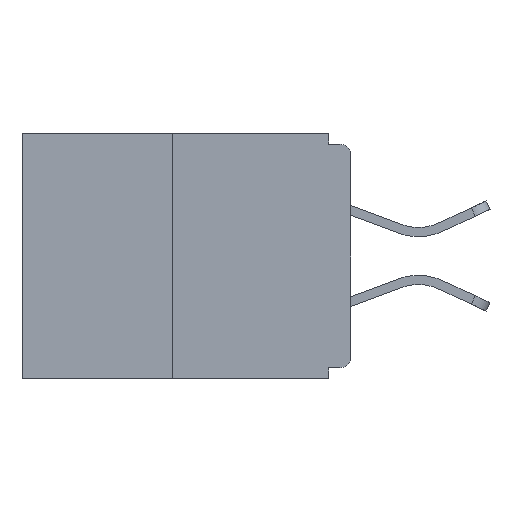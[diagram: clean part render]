
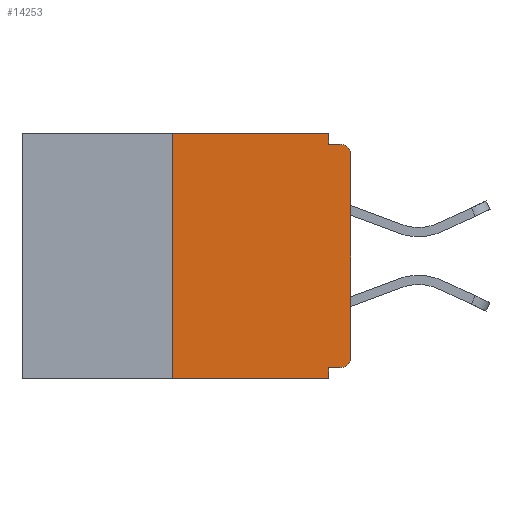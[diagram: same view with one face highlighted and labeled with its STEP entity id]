
A CAD part, left-side view. The second image highlights one B-rep face of the part: STEP entity #14253.
In plain terms, the highlighted planar face has unit normal (-1, 0, 0).
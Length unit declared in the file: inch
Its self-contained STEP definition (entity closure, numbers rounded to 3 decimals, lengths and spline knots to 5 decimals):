
#59 = VERTEX_POINT ( 'NONE', #584 ) ;
#227 = VECTOR ( 'NONE', #20103, 39.37008 ) ;
#247 = DIRECTION ( 'NONE',  ( 0., 0., -1. ) ) ;
#301 = VECTOR ( 'NONE', #11030, 39.37008 ) ;
#584 = CARTESIAN_POINT ( 'NONE',  ( 0., 0., -0.03 ) ) ;
#733 = DIRECTION ( 'NONE',  ( 0., 0., 1. ) ) ;
#843 = VERTEX_POINT ( 'NONE', #1978 ) ;
#1314 = CARTESIAN_POINT ( 'NONE',  ( 0., 0.25, -0.343 ) ) ;
#1721 = DIRECTION ( 'NONE',  ( 0., 0., -1. ) ) ;
#1902 = DIRECTION ( 'NONE',  ( -1., 0., 0. ) ) ;
#1978 = CARTESIAN_POINT ( 'NONE',  ( 0., 0.031, -0.015 ) ) ;
#2137 = VECTOR ( 'NONE', #18872, 39.37008 ) ;
#2547 = VECTOR ( 'NONE', #5426, 39.37008 ) ;
#2620 = LINE ( 'NONE', #13491, #2137 ) ;
#2725 = CARTESIAN_POINT ( 'NONE',  ( 0., 0.031, 0. ) ) ;
#2933 = VERTEX_POINT ( 'NONE', #2725 ) ;
#3170 = LINE ( 'NONE', #14234, #20039 ) ;
#3795 = CARTESIAN_POINT ( 'NONE',  ( 0., 0.46, -0.343 ) ) ;
#3861 = ORIENTED_EDGE ( 'NONE', *, *, #11914, .F. ) ;
#3948 = VERTEX_POINT ( 'NONE', #10906 ) ;
#4405 = VERTEX_POINT ( 'NONE', #1314 ) ;
#4603 = EDGE_CURVE ( 'NONE', #4405, #11084, #15252, .T. ) ;
#4898 = LINE ( 'NONE', #18395, #9749 ) ;
#4911 = CIRCLE ( 'NONE', #20896, 0.015 ) ;
#5142 = CARTESIAN_POINT ( 'NONE',  ( 0., 0.46, 0. ) ) ;
#5207 = DIRECTION ( 'NONE',  ( 0., 0., -1. ) ) ;
#5395 = ORIENTED_EDGE ( 'NONE', *, *, #4603, .T. ) ;
#5426 = DIRECTION ( 'NONE',  ( 0., -1., 0. ) ) ;
#5513 = CARTESIAN_POINT ( 'NONE',  ( 0., 0.25, 0. ) ) ;
#5656 = CARTESIAN_POINT ( 'NONE',  ( 0., 0.031, -0.343 ) ) ;
#5693 = FACE_OUTER_BOUND ( 'NONE', #15915, .T. ) ;
#5942 = VERTEX_POINT ( 'NONE', #11669 ) ;
#6926 = LINE ( 'NONE', #19632, #7389 ) ;
#6938 = LINE ( 'NONE', #9232, #301 ) ;
#7042 = VERTEX_POINT ( 'NONE', #15984 ) ;
#7389 = VECTOR ( 'NONE', #1721, 39.37008 ) ;
#8378 = LINE ( 'NONE', #18496, #227 ) ;
#8554 = EDGE_CURVE ( 'NONE', #10093, #2933, #3170, .T. ) ;
#8970 = EDGE_CURVE ( 'NONE', #7042, #5942, #4911, .T. ) ;
#9146 = AXIS2_PLACEMENT_3D ( 'NONE', #16800, #1902, #247 ) ;
#9232 = CARTESIAN_POINT ( 'NONE',  ( 0., 0.031, -0.343 ) ) ;
#9235 = EDGE_CURVE ( 'NONE', #843, #3948, #2620, .T. ) ;
#9749 = VECTOR ( 'NONE', #19874, 39.37008 ) ;
#10093 = VERTEX_POINT ( 'NONE', #5513 ) ;
#10235 = ORIENTED_EDGE ( 'NONE', *, *, #9235, .F. ) ;
#10802 = AXIS2_PLACEMENT_3D ( 'NONE', #5142, #18184, #5207 ) ;
#10906 = CARTESIAN_POINT ( 'NONE',  ( 0., 0.015, -0.015 ) ) ;
#11030 = DIRECTION ( 'NONE',  ( 0., 0., -1. ) ) ;
#11083 = DIRECTION ( 'NONE',  ( -1., 0., 0. ) ) ;
#11084 = VERTEX_POINT ( 'NONE', #5656 ) ;
#11669 = CARTESIAN_POINT ( 'NONE',  ( 0., 0., -0.313 ) ) ;
#11702 = ORIENTED_EDGE ( 'NONE', *, *, #14979, .F. ) ;
#11914 = EDGE_CURVE ( 'NONE', #7042, #20059, #8378, .T. ) ;
#12348 = CIRCLE ( 'NONE', #9146, 0.015 ) ;
#12476 = DIRECTION ( 'NONE',  ( 0., -1., 0. ) ) ;
#13239 = ORIENTED_EDGE ( 'NONE', *, *, #16351, .F. ) ;
#13345 = ORIENTED_EDGE ( 'NONE', *, *, #8970, .T. ) ;
#13399 = EDGE_CURVE ( 'NONE', #59, #3948, #12348, .T. ) ;
#13491 = CARTESIAN_POINT ( 'NONE',  ( 0., 0., -0.015 ) ) ;
#13631 = ORIENTED_EDGE ( 'NONE', *, *, #18291, .F. ) ;
#14122 = ORIENTED_EDGE ( 'NONE', *, *, #13399, .T. ) ;
#14234 = CARTESIAN_POINT ( 'NONE',  ( 0., 0.46, 0. ) ) ;
#14253 = ADVANCED_FACE ( 'NONE', ( #5693 ), #16646, .F. ) ;
#14979 = EDGE_CURVE ( 'NONE', #4405, #10093, #4898, .T. ) ;
#15049 = ORIENTED_EDGE ( 'NONE', *, *, #21071, .T. ) ;
#15252 = LINE ( 'NONE', #3795, #2547 ) ;
#15915 = EDGE_LOOP ( 'NONE', ( #21138, #11702, #5395, #13631, #3861, #13345, #15049, #14122, #10235, #13239 ) ) ;
#15984 = CARTESIAN_POINT ( 'NONE',  ( 0., 0.015, -0.328 ) ) ;
#16038 = DIRECTION ( 'NONE',  ( 0., 0., -1. ) ) ;
#16351 = EDGE_CURVE ( 'NONE', #2933, #843, #6926, .T. ) ;
#16646 = PLANE ( 'NONE',  #10802 ) ;
#16800 = CARTESIAN_POINT ( 'NONE',  ( 0., 0.015, -0.03 ) ) ;
#17727 = VECTOR ( 'NONE', #733, 39.37008 ) ;
#18184 = DIRECTION ( 'NONE',  ( 1., 0., 0. ) ) ;
#18263 = LINE ( 'NONE', #20018, #17727 ) ;
#18291 = EDGE_CURVE ( 'NONE', #20059, #11084, #6938, .T. ) ;
#18395 = CARTESIAN_POINT ( 'NONE',  ( 0., 0.25, 0. ) ) ;
#18496 = CARTESIAN_POINT ( 'NONE',  ( 0., 0., -0.328 ) ) ;
#18872 = DIRECTION ( 'NONE',  ( 0., -1., 0. ) ) ;
#19267 = CARTESIAN_POINT ( 'NONE',  ( 0., 0.015, -0.313 ) ) ;
#19632 = CARTESIAN_POINT ( 'NONE',  ( 0., 0.031, 0. ) ) ;
#19874 = DIRECTION ( 'NONE',  ( 0., 0., 1. ) ) ;
#20018 = CARTESIAN_POINT ( 'NONE',  ( 0., 0., 0. ) ) ;
#20039 = VECTOR ( 'NONE', #12476, 39.37008 ) ;
#20059 = VERTEX_POINT ( 'NONE', #20575 ) ;
#20103 = DIRECTION ( 'NONE',  ( 0., 1., 0. ) ) ;
#20575 = CARTESIAN_POINT ( 'NONE',  ( 0., 0.031, -0.328 ) ) ;
#20896 = AXIS2_PLACEMENT_3D ( 'NONE', #19267, #11083, #16038 ) ;
#21071 = EDGE_CURVE ( 'NONE', #5942, #59, #18263, .T. ) ;
#21138 = ORIENTED_EDGE ( 'NONE', *, *, #8554, .F. ) ;
